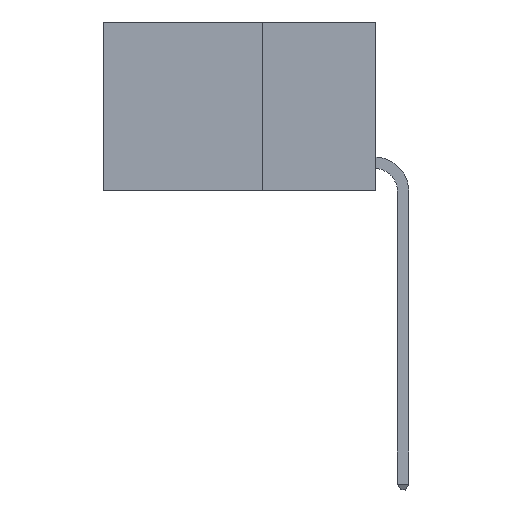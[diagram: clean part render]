
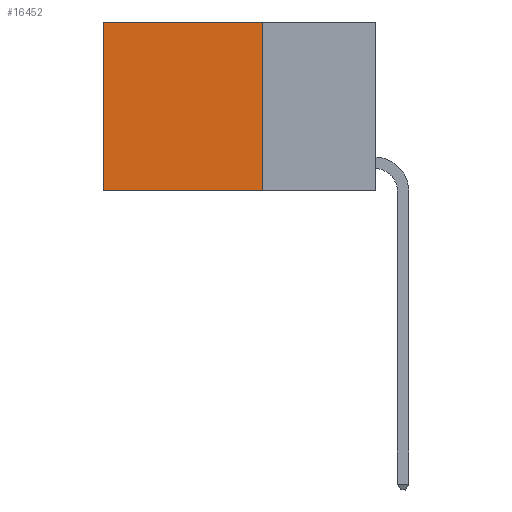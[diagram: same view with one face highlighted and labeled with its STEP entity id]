
A CAD part, left-side view. The second image highlights one B-rep face of the part: STEP entity #16452.
In plain terms, the highlighted planar face has unit normal (-1, 0, 0).
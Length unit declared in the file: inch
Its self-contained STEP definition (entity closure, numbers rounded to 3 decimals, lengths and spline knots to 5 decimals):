
#2018 = EDGE_CURVE ( 'NONE', #4473, #7613, #10830, .T. ) ;
#2227 = DIRECTION ( 'NONE',  ( 0., 1., 0. ) ) ;
#3579 = VECTOR ( 'NONE', #16627, 39.37008 ) ;
#4179 = CARTESIAN_POINT ( 'NONE',  ( 0.2625, 0.25, -0.37 ) ) ;
#4376 = AXIS2_PLACEMENT_3D ( 'NONE', #8653, #20033, #10294 ) ;
#4473 = VERTEX_POINT ( 'NONE', #8205 ) ;
#4772 = DIRECTION ( 'NONE',  ( 0., 1., 0. ) ) ;
#6859 = CARTESIAN_POINT ( 'NONE',  ( 0.2625, 0.6, -0.37 ) ) ;
#7286 = EDGE_LOOP ( 'NONE', ( #7701, #10689, #8809, #20971 ) ) ;
#7613 = VERTEX_POINT ( 'NONE', #6859 ) ;
#7701 = ORIENTED_EDGE ( 'NONE', *, *, #15406, .T. ) ;
#7830 = CARTESIAN_POINT ( 'NONE',  ( 0.2625, 0.25, 0. ) ) ;
#8205 = CARTESIAN_POINT ( 'NONE',  ( 0.2625, 0.25, -0.37 ) ) ;
#8653 = CARTESIAN_POINT ( 'NONE',  ( 0.2625, 0.25, 0. ) ) ;
#8809 = ORIENTED_EDGE ( 'NONE', *, *, #10181, .F. ) ;
#9157 = VERTEX_POINT ( 'NONE', #7830 ) ;
#10181 = EDGE_CURVE ( 'NONE', #9157, #4473, #11022, .T. ) ;
#10294 = DIRECTION ( 'NONE',  ( 0., 0., -1. ) ) ;
#10689 = ORIENTED_EDGE ( 'NONE', *, *, #2018, .F. ) ;
#10830 = LINE ( 'NONE', #4179, #14683 ) ;
#11022 = LINE ( 'NONE', #20405, #19179 ) ;
#12355 = LINE ( 'NONE', #14973, #3579 ) ;
#13598 = EDGE_CURVE ( 'NONE', #9157, #19826, #18798, .T. ) ;
#14466 = VECTOR ( 'NONE', #2227, 39.37008 ) ;
#14683 = VECTOR ( 'NONE', #4772, 39.37008 ) ;
#14973 = CARTESIAN_POINT ( 'NONE',  ( 0.2625, 0.6, 0. ) ) ;
#15406 = EDGE_CURVE ( 'NONE', #19826, #7613, #12355, .T. ) ;
#16452 = ADVANCED_FACE ( 'NONE', ( #18417 ), #18411, .F. ) ;
#16627 = DIRECTION ( 'NONE',  ( 0., 0., -1. ) ) ;
#18208 = CARTESIAN_POINT ( 'NONE',  ( 0.2625, 0.6, 0. ) ) ;
#18411 = PLANE ( 'NONE',  #4376 ) ;
#18417 = FACE_OUTER_BOUND ( 'NONE', #7286, .T. ) ;
#18597 = CARTESIAN_POINT ( 'NONE',  ( 0.2625, 0.25, 0. ) ) ;
#18798 = LINE ( 'NONE', #18597, #14466 ) ;
#18867 = DIRECTION ( 'NONE',  ( 0., 0., -1. ) ) ;
#19179 = VECTOR ( 'NONE', #18867, 39.37008 ) ;
#19826 = VERTEX_POINT ( 'NONE', #18208 ) ;
#20033 = DIRECTION ( 'NONE',  ( 1., 0., 0. ) ) ;
#20405 = CARTESIAN_POINT ( 'NONE',  ( 0.2625, 0.25, 0. ) ) ;
#20971 = ORIENTED_EDGE ( 'NONE', *, *, #13598, .T. ) ;
